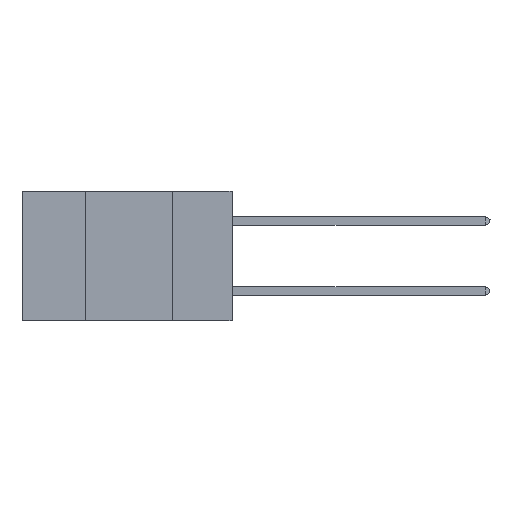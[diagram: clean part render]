
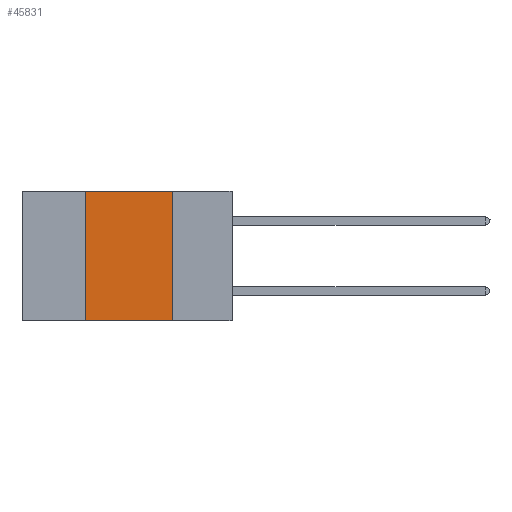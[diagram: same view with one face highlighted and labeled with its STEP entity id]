
A CAD part, left-side view. The second image highlights one B-rep face of the part: STEP entity #45831.
In plain terms, the highlighted planar face has unit normal (-1, 0, 0).
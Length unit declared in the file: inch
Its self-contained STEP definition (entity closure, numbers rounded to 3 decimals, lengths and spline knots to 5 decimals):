
#281 = CARTESIAN_POINT ( 'NONE',  ( 0., 0.17, 0. ) ) ;
#845 = AXIS2_PLACEMENT_3D ( 'NONE', #42409, #20674, #6208 ) ;
#4633 = VECTOR ( 'NONE', #31494, 39.37008 ) ;
#5979 = PLANE ( 'NONE',  #845 ) ;
#6208 = DIRECTION ( 'NONE',  ( 0., 0., -1. ) ) ;
#10739 = VERTEX_POINT ( 'NONE', #20855 ) ;
#12439 = DIRECTION ( 'NONE',  ( 0., 0., -1. ) ) ;
#12467 = CARTESIAN_POINT ( 'NONE',  ( 0., 0.6, 0. ) ) ;
#12920 = CARTESIAN_POINT ( 'NONE',  ( 0., 0.17, 0. ) ) ;
#13358 = DIRECTION ( 'NONE',  ( 0., -1., 0. ) ) ;
#14144 = ORIENTED_EDGE ( 'NONE', *, *, #27606, .F. ) ;
#14528 = VERTEX_POINT ( 'NONE', #28922 ) ;
#17994 = VECTOR ( 'NONE', #34763, 39.37008 ) ;
#18094 = EDGE_LOOP ( 'NONE', ( #41853, #14144, #23215, #21862 ) ) ;
#19428 = LINE ( 'NONE', #12920, #28477 ) ;
#19700 = LINE ( 'NONE', #12467, #37529 ) ;
#20674 = DIRECTION ( 'NONE',  ( 1., 0., 0. ) ) ;
#20855 = CARTESIAN_POINT ( 'NONE',  ( 0., 0.17, -0.37 ) ) ;
#21862 = ORIENTED_EDGE ( 'NONE', *, *, #44410, .T. ) ;
#23215 = ORIENTED_EDGE ( 'NONE', *, *, #38980, .F. ) ;
#26401 = VERTEX_POINT ( 'NONE', #41594 ) ;
#27606 = EDGE_CURVE ( 'NONE', #14528, #46444, #19700, .T. ) ;
#28477 = VECTOR ( 'NONE', #12439, 39.37008 ) ;
#28922 = CARTESIAN_POINT ( 'NONE',  ( 0., 0.42, 0. ) ) ;
#31494 = DIRECTION ( 'NONE',  ( 0., -1., 0. ) ) ;
#33811 = LINE ( 'NONE', #41759, #17994 ) ;
#34763 = DIRECTION ( 'NONE',  ( 0., 0., 1. ) ) ;
#37529 = VECTOR ( 'NONE', #13358, 39.37008 ) ;
#37774 = CARTESIAN_POINT ( 'NONE',  ( 0., 0.6, -0.37 ) ) ;
#38980 = EDGE_CURVE ( 'NONE', #26401, #14528, #33811, .T. ) ;
#39030 = FACE_OUTER_BOUND ( 'NONE', #18094, .T. ) ;
#41394 = LINE ( 'NONE', #37774, #4633 ) ;
#41594 = CARTESIAN_POINT ( 'NONE',  ( 0., 0.42, -0.37 ) ) ;
#41759 = CARTESIAN_POINT ( 'NONE',  ( 0., 0.42, 0. ) ) ;
#41853 = ORIENTED_EDGE ( 'NONE', *, *, #44298, .F. ) ;
#42409 = CARTESIAN_POINT ( 'NONE',  ( 0., 0.6, 0. ) ) ;
#44298 = EDGE_CURVE ( 'NONE', #46444, #10739, #19428, .T. ) ;
#44410 = EDGE_CURVE ( 'NONE', #26401, #10739, #41394, .T. ) ;
#45831 = ADVANCED_FACE ( 'NONE', ( #39030 ), #5979, .F. ) ;
#46444 = VERTEX_POINT ( 'NONE', #281 ) ;
